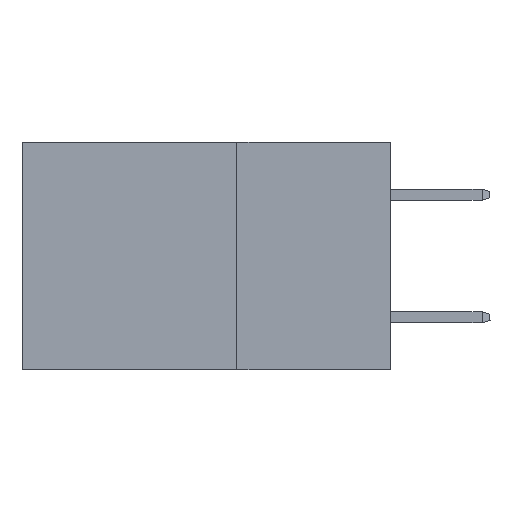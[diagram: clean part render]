
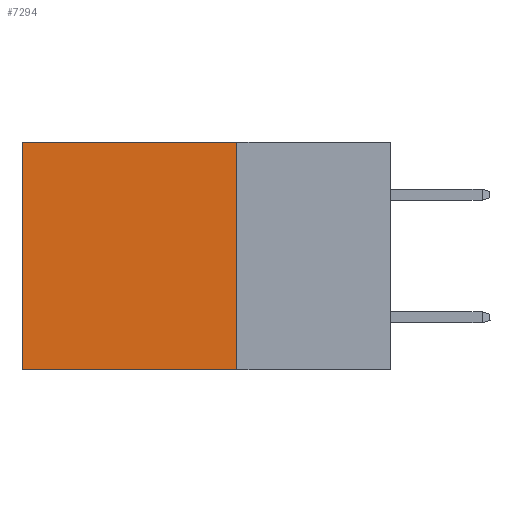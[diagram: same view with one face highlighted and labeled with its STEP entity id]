
A CAD part, left-side view. The second image highlights one B-rep face of the part: STEP entity #7294.
In plain terms, the highlighted planar face has unit normal (-1, 0, 0).
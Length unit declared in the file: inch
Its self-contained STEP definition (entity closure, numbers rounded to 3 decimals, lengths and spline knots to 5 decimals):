
#1546 = CARTESIAN_POINT ( 'NONE',  ( 0.2875, 0.25, 0. ) ) ;
#1961 = DIRECTION ( 'NONE',  ( 0., 0., -1. ) ) ;
#2187 = DIRECTION ( 'NONE',  ( 0., 1., 0. ) ) ;
#2606 = EDGE_CURVE ( 'NONE', #11300, #9130, #8081, .T. ) ;
#3506 = ORIENTED_EDGE ( 'NONE', *, *, #2606, .T. ) ;
#3607 = CARTESIAN_POINT ( 'NONE',  ( 0.2875, 0.25, -0.37 ) ) ;
#3678 = EDGE_CURVE ( 'NONE', #3789, #4139, #12455, .T. ) ;
#3789 = VERTEX_POINT ( 'NONE', #8147 ) ;
#4139 = VERTEX_POINT ( 'NONE', #3607 ) ;
#4616 = CARTESIAN_POINT ( 'NONE',  ( 0.2875, 0.25, -0.37 ) ) ;
#4666 = PLANE ( 'NONE',  #8067 ) ;
#4937 = DIRECTION ( 'NONE',  ( 0., 0., -1. ) ) ;
#5439 = ORIENTED_EDGE ( 'NONE', *, *, #8629, .T. ) ;
#5851 = VECTOR ( 'NONE', #5871, 39.37008 ) ;
#5871 = DIRECTION ( 'NONE',  ( 0., 1., 0. ) ) ;
#5973 = EDGE_CURVE ( 'NONE', #4139, #9130, #9478, .T. ) ;
#6000 = LINE ( 'NONE', #10758, #5851 ) ;
#6221 = VECTOR ( 'NONE', #2187, 39.37008 ) ;
#6432 = EDGE_LOOP ( 'NONE', ( #3506, #12646, #12028, #5439 ) ) ;
#7294 = ADVANCED_FACE ( 'NONE', ( #11338 ), #4666, .F. ) ;
#7710 = CARTESIAN_POINT ( 'NONE',  ( 0.2875, 0.6, -0.37 ) ) ;
#8067 = AXIS2_PLACEMENT_3D ( 'NONE', #1546, #11407, #10507 ) ;
#8081 = LINE ( 'NONE', #11991, #12141 ) ;
#8122 = CARTESIAN_POINT ( 'NONE',  ( 0.2875, 0.6, 0. ) ) ;
#8147 = CARTESIAN_POINT ( 'NONE',  ( 0.2875, 0.25, 0. ) ) ;
#8629 = EDGE_CURVE ( 'NONE', #3789, #11300, #6000, .T. ) ;
#9130 = VERTEX_POINT ( 'NONE', #7710 ) ;
#9478 = LINE ( 'NONE', #4616, #6221 ) ;
#9504 = VECTOR ( 'NONE', #1961, 39.37008 ) ;
#9693 = CARTESIAN_POINT ( 'NONE',  ( 0.2875, 0.25, 0. ) ) ;
#10507 = DIRECTION ( 'NONE',  ( 0., 0., -1. ) ) ;
#10758 = CARTESIAN_POINT ( 'NONE',  ( 0.2875, 0.25, 0. ) ) ;
#11300 = VERTEX_POINT ( 'NONE', #8122 ) ;
#11338 = FACE_OUTER_BOUND ( 'NONE', #6432, .T. ) ;
#11407 = DIRECTION ( 'NONE',  ( 1., 0., 0. ) ) ;
#11991 = CARTESIAN_POINT ( 'NONE',  ( 0.2875, 0.6, 0. ) ) ;
#12028 = ORIENTED_EDGE ( 'NONE', *, *, #3678, .F. ) ;
#12141 = VECTOR ( 'NONE', #4937, 39.37008 ) ;
#12455 = LINE ( 'NONE', #9693, #9504 ) ;
#12646 = ORIENTED_EDGE ( 'NONE', *, *, #5973, .F. ) ;
